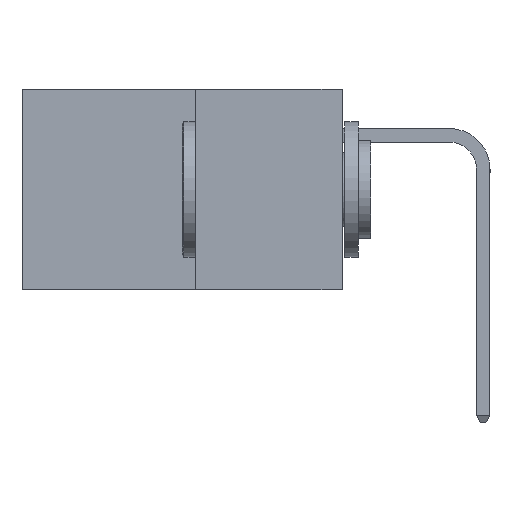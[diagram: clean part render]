
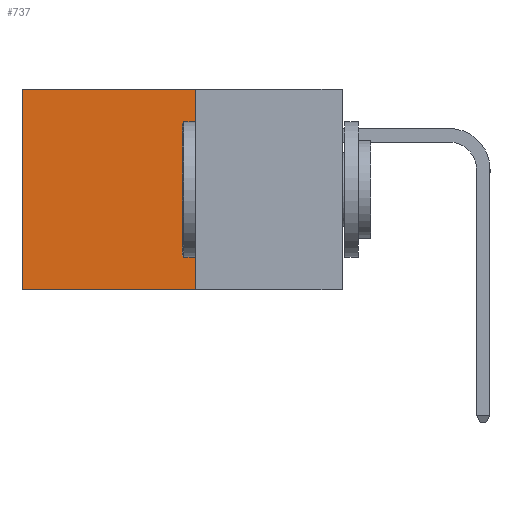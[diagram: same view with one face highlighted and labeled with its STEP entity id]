
A CAD part, left-side view. The second image highlights one B-rep face of the part: STEP entity #737.
In plain terms, the highlighted planar face has unit normal (-1, 0, 0).
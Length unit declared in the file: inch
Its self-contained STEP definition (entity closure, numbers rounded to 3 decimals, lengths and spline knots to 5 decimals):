
#76 = DIRECTION ( 'NONE',  ( 0., 0., -1. ) ) ;
#737 = ADVANCED_FACE ( 'NONE', ( #2295 ), #8939, .F. ) ;
#1032 = DIRECTION ( 'NONE',  ( 0., 0., -1. ) ) ;
#1857 = ORIENTED_EDGE ( 'NONE', *, *, #2145, .F. ) ;
#2145 = EDGE_CURVE ( 'NONE', #4677, #10481, #7125, .T. ) ;
#2295 = FACE_OUTER_BOUND ( 'NONE', #9822, .T. ) ;
#2580 = CARTESIAN_POINT ( 'NONE',  ( 0.277, 0.27, 0. ) ) ;
#2605 = DIRECTION ( 'NONE',  ( 0., 1., 0. ) ) ;
#2856 = CARTESIAN_POINT ( 'NONE',  ( 0.277, 0.59, 0. ) ) ;
#2967 = LINE ( 'NONE', #4593, #10032 ) ;
#3066 = VERTEX_POINT ( 'NONE', #3622 ) ;
#3125 = EDGE_CURVE ( 'NONE', #3066, #10815, #11440, .T. ) ;
#3583 = VECTOR ( 'NONE', #2605, 39.37008 ) ;
#3622 = CARTESIAN_POINT ( 'NONE',  ( 0.277, 0.27, 0. ) ) ;
#4020 = ORIENTED_EDGE ( 'NONE', *, *, #11682, .T. ) ;
#4312 = ORIENTED_EDGE ( 'NONE', *, *, #9040, .F. ) ;
#4593 = CARTESIAN_POINT ( 'NONE',  ( 0.277, 0.59, -0.37 ) ) ;
#4677 = VERTEX_POINT ( 'NONE', #5381 ) ;
#4875 = DIRECTION ( 'NONE',  ( 0., 1., 0. ) ) ;
#5381 = CARTESIAN_POINT ( 'NONE',  ( 0.277, 0.27, -0.37 ) ) ;
#6353 = AXIS2_PLACEMENT_3D ( 'NONE', #8663, #8647, #76 ) ;
#6462 = CARTESIAN_POINT ( 'NONE',  ( 0.277, 0.27, -0.37 ) ) ;
#7125 = LINE ( 'NONE', #6462, #11587 ) ;
#8647 = DIRECTION ( 'NONE',  ( 1., 0., 0. ) ) ;
#8663 = CARTESIAN_POINT ( 'NONE',  ( 0.277, 0.27, -0.37 ) ) ;
#8939 = PLANE ( 'NONE',  #6353 ) ;
#9040 = EDGE_CURVE ( 'NONE', #3066, #4677, #9476, .T. ) ;
#9198 = ORIENTED_EDGE ( 'NONE', *, *, #3125, .T. ) ;
#9476 = LINE ( 'NONE', #10237, #11277 ) ;
#9822 = EDGE_LOOP ( 'NONE', ( #4020, #1857, #4312, #9198 ) ) ;
#10032 = VECTOR ( 'NONE', #10098, 39.37008 ) ;
#10098 = DIRECTION ( 'NONE',  ( 0., 0., -1. ) ) ;
#10237 = CARTESIAN_POINT ( 'NONE',  ( 0.277, 0.27, -0.37 ) ) ;
#10481 = VERTEX_POINT ( 'NONE', #10610 ) ;
#10610 = CARTESIAN_POINT ( 'NONE',  ( 0.277, 0.59, -0.37 ) ) ;
#10815 = VERTEX_POINT ( 'NONE', #2856 ) ;
#11277 = VECTOR ( 'NONE', #1032, 39.37008 ) ;
#11440 = LINE ( 'NONE', #2580, #3583 ) ;
#11587 = VECTOR ( 'NONE', #4875, 39.37008 ) ;
#11682 = EDGE_CURVE ( 'NONE', #10815, #10481, #2967, .T. ) ;
